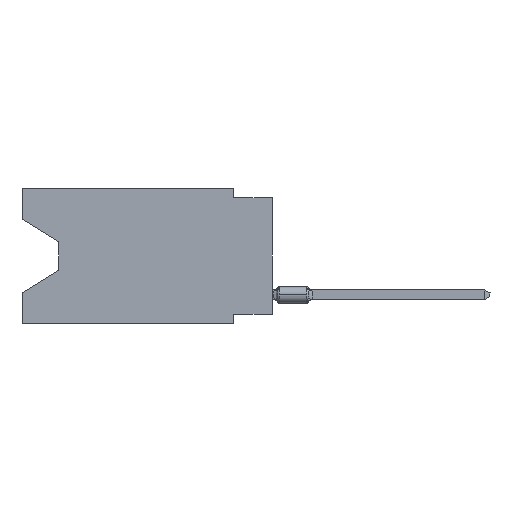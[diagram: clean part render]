
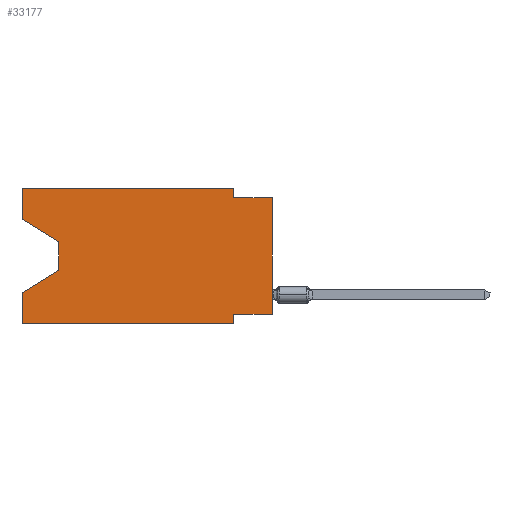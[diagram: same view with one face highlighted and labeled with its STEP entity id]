
A CAD part, left-side view. The second image highlights one B-rep face of the part: STEP entity #33177.
In plain terms, the highlighted planar face has unit normal (-1, 0, 0).
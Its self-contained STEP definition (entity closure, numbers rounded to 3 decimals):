
#1602 = DIRECTION ( 'NONE',  ( 0., -1., 0. ) ) ;
#1944 = VECTOR ( 'NONE', #44713, 1000. ) ;
#2143 = EDGE_CURVE ( 'NONE', #43332, #27330, #9998, .T. ) ;
#2267 = CARTESIAN_POINT ( 'NONE',  ( 0., 16.383, 0. ) ) ;
#3115 = CARTESIAN_POINT ( 'NONE',  ( 0., 0., 0. ) ) ;
#3439 = LINE ( 'NONE', #3115, #26732 ) ;
#3528 = LINE ( 'NONE', #4527, #19817 ) ;
#3688 = LINE ( 'NONE', #44951, #56521 ) ;
#4106 = CARTESIAN_POINT ( 'NONE',  ( 0., 2.54, -8.89 ) ) ;
#4283 = EDGE_CURVE ( 'NONE', #7152, #18162, #38471, .T. ) ;
#4397 = ORIENTED_EDGE ( 'NONE', *, *, #9662, .T. ) ;
#4499 = CARTESIAN_POINT ( 'NONE',  ( 0., 16.383, -2.038 ) ) ;
#4527 = CARTESIAN_POINT ( 'NONE',  ( 0., 16.383, -8.89 ) ) ;
#4558 = LINE ( 'NONE', #25063, #26599 ) ;
#4727 = VERTEX_POINT ( 'NONE', #9156 ) ;
#7152 = VERTEX_POINT ( 'NONE', #53348 ) ;
#8339 = VECTOR ( 'NONE', #32095, 1000. ) ;
#9156 = CARTESIAN_POINT ( 'NONE',  ( 0., 2.54, -8.255 ) ) ;
#9252 = CARTESIAN_POINT ( 'NONE',  ( 0., 0., -0.635 ) ) ;
#9297 = CARTESIAN_POINT ( 'NONE',  ( 0., 2.54, -0.635 ) ) ;
#9662 = EDGE_CURVE ( 'NONE', #16481, #61168, #3528, .T. ) ;
#9977 = ORIENTED_EDGE ( 'NONE', *, *, #35766, .T. ) ;
#9998 = LINE ( 'NONE', #2267, #60098 ) ;
#10517 = EDGE_CURVE ( 'NONE', #23405, #7152, #3688, .T. ) ;
#11516 = ORIENTED_EDGE ( 'NONE', *, *, #2143, .F. ) ;
#11592 = CARTESIAN_POINT ( 'NONE',  ( 0., 2.54, 0. ) ) ;
#12261 = EDGE_CURVE ( 'NONE', #16481, #41667, #29985, .T. ) ;
#13927 = DIRECTION ( 'NONE',  ( 0., -1., 0. ) ) ;
#14461 = CARTESIAN_POINT ( 'NONE',  ( 0., 16.383, 0. ) ) ;
#15764 = CARTESIAN_POINT ( 'NONE',  ( 0., 16.383, 0. ) ) ;
#16200 = VERTEX_POINT ( 'NONE', #16506 ) ;
#16465 = CARTESIAN_POINT ( 'NONE',  ( 0., 2.54, 0. ) ) ;
#16481 = VERTEX_POINT ( 'NONE', #57346 ) ;
#16506 = CARTESIAN_POINT ( 'NONE',  ( 0., 0., -8.255 ) ) ;
#17152 = EDGE_CURVE ( 'NONE', #4727, #61168, #63625, .T. ) ;
#17664 = CARTESIAN_POINT ( 'NONE',  ( 0., 2.54, -8.89 ) ) ;
#18162 = VERTEX_POINT ( 'NONE', #34395 ) ;
#18489 = EDGE_CURVE ( 'NONE', #16200, #52094, #3439, .T. ) ;
#18551 = DIRECTION ( 'NONE',  ( 0., 0., 1. ) ) ;
#18642 = VECTOR ( 'NONE', #23090, 1000. ) ;
#18660 = CARTESIAN_POINT ( 'NONE',  ( 0., 13.97, -3.505 ) ) ;
#19358 = DIRECTION ( 'NONE',  ( 1., 0., 0. ) ) ;
#19566 = CARTESIAN_POINT ( 'NONE',  ( 0., 16.383, 0. ) ) ;
#19745 = ORIENTED_EDGE ( 'NONE', *, *, #10517, .T. ) ;
#19817 = VECTOR ( 'NONE', #13927, 1000. ) ;
#20901 = CARTESIAN_POINT ( 'NONE',  ( 0., 16.383, -6.852 ) ) ;
#22714 = ORIENTED_EDGE ( 'NONE', *, *, #18489, .T. ) ;
#22743 = DIRECTION ( 'NONE',  ( 0., 0., -1. ) ) ;
#22896 = VECTOR ( 'NONE', #22743, 1000. ) ;
#23090 = DIRECTION ( 'NONE',  ( 0., -1., 0. ) ) ;
#23405 = VERTEX_POINT ( 'NONE', #4499 ) ;
#23415 = FACE_OUTER_BOUND ( 'NONE', #63626, .T. ) ;
#23509 = ORIENTED_EDGE ( 'NONE', *, *, #17152, .F. ) ;
#23847 = EDGE_CURVE ( 'NONE', #23405, #43332, #44348, .T. ) ;
#24394 = PLANE ( 'NONE',  #42597 ) ;
#25063 = CARTESIAN_POINT ( 'NONE',  ( 0., 13.97, -5.385 ) ) ;
#26599 = VECTOR ( 'NONE', #55898, 1000. ) ;
#26732 = VECTOR ( 'NONE', #18551, 1000. ) ;
#27330 = VERTEX_POINT ( 'NONE', #16465 ) ;
#28445 = LINE ( 'NONE', #59294, #18642 ) ;
#29985 = LINE ( 'NONE', #19566, #1944 ) ;
#32095 = DIRECTION ( 'NONE',  ( 0., 0., -1. ) ) ;
#32648 = LINE ( 'NONE', #32978, #41595 ) ;
#32978 = CARTESIAN_POINT ( 'NONE',  ( 0., 0., -8.255 ) ) ;
#33105 = DIRECTION ( 'NONE',  ( 0., 0., -1. ) ) ;
#33177 = ADVANCED_FACE ( 'NONE', ( #23415 ), #24394, .F. ) ;
#34395 = CARTESIAN_POINT ( 'NONE',  ( 0., 13.97, -5.385 ) ) ;
#35766 = EDGE_CURVE ( 'NONE', #18162, #41667, #4558, .T. ) ;
#36464 = EDGE_CURVE ( 'NONE', #16200, #4727, #32648, .T. ) ;
#37087 = LINE ( 'NONE', #11592, #8339 ) ;
#38471 = LINE ( 'NONE', #18660, #22896 ) ;
#39125 = VECTOR ( 'NONE', #65814, 1000. ) ;
#39924 = DIRECTION ( 'NONE',  ( 0., -0.855, -0.519 ) ) ;
#41595 = VECTOR ( 'NONE', #53433, 1000. ) ;
#41667 = VERTEX_POINT ( 'NONE', #20901 ) ;
#42593 = ORIENTED_EDGE ( 'NONE', *, *, #23847, .F. ) ;
#42597 = AXIS2_PLACEMENT_3D ( 'NONE', #65311, #19358, #64319 ) ;
#43332 = VERTEX_POINT ( 'NONE', #15764 ) ;
#44288 = EDGE_CURVE ( 'NONE', #27330, #53084, #37087, .T. ) ;
#44348 = LINE ( 'NONE', #14461, #39125 ) ;
#44713 = DIRECTION ( 'NONE',  ( 0., 0., 1. ) ) ;
#44951 = CARTESIAN_POINT ( 'NONE',  ( 0., 16.383, -2.038 ) ) ;
#45458 = ORIENTED_EDGE ( 'NONE', *, *, #36464, .F. ) ;
#48951 = ORIENTED_EDGE ( 'NONE', *, *, #58787, .F. ) ;
#52094 = VERTEX_POINT ( 'NONE', #9252 ) ;
#53084 = VERTEX_POINT ( 'NONE', #9297 ) ;
#53348 = CARTESIAN_POINT ( 'NONE',  ( 0., 13.97, -3.505 ) ) ;
#53433 = DIRECTION ( 'NONE',  ( 0., 1., 0. ) ) ;
#54261 = ORIENTED_EDGE ( 'NONE', *, *, #44288, .F. ) ;
#55784 = VECTOR ( 'NONE', #33105, 1000. ) ;
#55898 = DIRECTION ( 'NONE',  ( 0., 0.855, -0.519 ) ) ;
#56521 = VECTOR ( 'NONE', #39924, 1000. ) ;
#57116 = ORIENTED_EDGE ( 'NONE', *, *, #4283, .T. ) ;
#57346 = CARTESIAN_POINT ( 'NONE',  ( 0., 16.383, -8.89 ) ) ;
#57765 = ORIENTED_EDGE ( 'NONE', *, *, #12261, .F. ) ;
#58787 = EDGE_CURVE ( 'NONE', #53084, #52094, #28445, .T. ) ;
#59294 = CARTESIAN_POINT ( 'NONE',  ( 0., 0., -0.635 ) ) ;
#60098 = VECTOR ( 'NONE', #1602, 1000. ) ;
#61168 = VERTEX_POINT ( 'NONE', #4106 ) ;
#63625 = LINE ( 'NONE', #17664, #55784 ) ;
#63626 = EDGE_LOOP ( 'NONE', ( #19745, #57116, #9977, #57765, #4397, #23509, #45458, #22714, #48951, #54261, #11516, #42593 ) ) ;
#64319 = DIRECTION ( 'NONE',  ( 0., 0., -1. ) ) ;
#65311 = CARTESIAN_POINT ( 'NONE',  ( 0., 16.383, 0. ) ) ;
#65814 = DIRECTION ( 'NONE',  ( 0., 0., 1. ) ) ;
